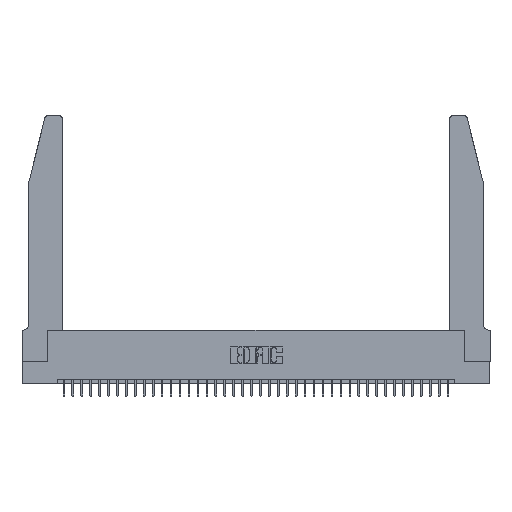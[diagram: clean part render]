
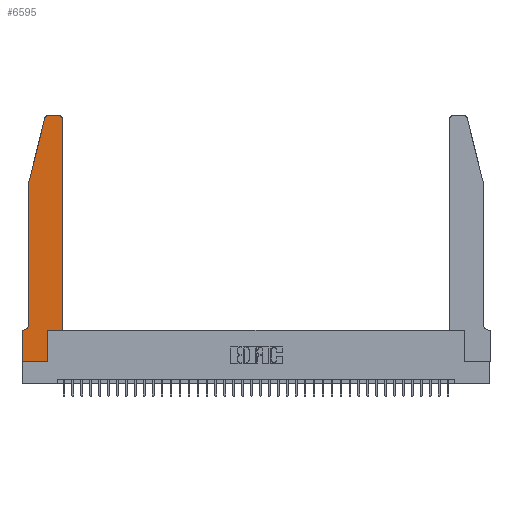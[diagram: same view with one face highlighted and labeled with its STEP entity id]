
A CAD part, top view. The second image highlights one B-rep face of the part: STEP entity #6595.
In plain terms, the highlighted planar face has unit normal (0, 0, 1).
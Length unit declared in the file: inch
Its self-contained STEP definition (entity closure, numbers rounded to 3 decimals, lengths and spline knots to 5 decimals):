
#118 = CARTESIAN_POINT ( 'NONE',  ( 0.2865, 0., 0.37 ) ) ;
#258 = EDGE_CURVE ( 'NONE', #8213, #38818, #25782, .T. ) ;
#737 = EDGE_CURVE ( 'NONE', #27138, #36192, #26523, .T. ) ;
#896 = DIRECTION ( 'NONE',  ( 0., 1., 0. ) ) ;
#1675 = DIRECTION ( 'NONE',  ( -1., 0., 0. ) ) ;
#2012 = CARTESIAN_POINT ( 'NONE',  ( 0.4505, 0.35, 0.37 ) ) ;
#2099 = CARTESIAN_POINT ( 'NONE',  ( 0.4205, 2.75, 0.37 ) ) ;
#3438 = AXIS2_PLACEMENT_3D ( 'NONE', #30439, #6475, #11615 ) ;
#3980 = DIRECTION ( 'NONE',  ( -1., 0., 0. ) ) ;
#4992 = EDGE_LOOP ( 'NONE', ( #22678, #20300, #11298, #25107, #38642, #12023, #14114, #24046, #18698, #20896, #29442, #15454 ) ) ;
#5937 = CIRCLE ( 'NONE', #3438, 0.03 ) ;
#6475 = DIRECTION ( 'NONE',  ( 0., 0., 1. ) ) ;
#6574 = DIRECTION ( 'NONE',  ( 0., 1., 0. ) ) ;
#6595 = ADVANCED_FACE ( 'NONE', ( #8096 ), #20915, .T. ) ;
#6707 = VERTEX_POINT ( 'NONE', #21108 ) ;
#6776 = CARTESIAN_POINT ( 'NONE',  ( 0.0055, 0.42, 0.37 ) ) ;
#6974 = DIRECTION ( 'NONE',  ( 0., 0., 1. ) ) ;
#7736 = VECTOR ( 'NONE', #33740, 39.37008 ) ;
#8096 = FACE_OUTER_BOUND ( 'NONE', #4992, .T. ) ;
#8213 = VERTEX_POINT ( 'NONE', #11500 ) ;
#8714 = CARTESIAN_POINT ( 'NONE',  ( 0., 0.35, 0.37 ) ) ;
#8911 = EDGE_CURVE ( 'NONE', #25903, #9559, #16449, .T. ) ;
#9214 = LINE ( 'NONE', #15298, #7736 ) ;
#9313 = CARTESIAN_POINT ( 'NONE',  ( 0.0755, 0.35, 0.37 ) ) ;
#9559 = VERTEX_POINT ( 'NONE', #15037 ) ;
#9956 = CARTESIAN_POINT ( 'NONE',  ( 0.284, 2.72, 0.37 ) ) ;
#10359 = CARTESIAN_POINT ( 'NONE',  ( 0.2865, 0.35, 0.37 ) ) ;
#10365 = VERTEX_POINT ( 'NONE', #38243 ) ;
#10992 = CARTESIAN_POINT ( 'NONE',  ( 0.4505, 2.72, 0.37 ) ) ;
#11298 = ORIENTED_EDGE ( 'NONE', *, *, #29453, .T. ) ;
#11379 = VECTOR ( 'NONE', #32501, 39.37008 ) ;
#11500 = CARTESIAN_POINT ( 'NONE',  ( 0.2865, 0.35, 0.37 ) ) ;
#11615 = DIRECTION ( 'NONE',  ( 1., 0., 0. ) ) ;
#11688 = CIRCLE ( 'NONE', #23052, 0.07 ) ;
#12023 = ORIENTED_EDGE ( 'NONE', *, *, #737, .T. ) ;
#13085 = EDGE_CURVE ( 'NONE', #20091, #8213, #27633, .T. ) ;
#13497 = AXIS2_PLACEMENT_3D ( 'NONE', #9956, #6974, #28169 ) ;
#14114 = ORIENTED_EDGE ( 'NONE', *, *, #36691, .T. ) ;
#15037 = CARTESIAN_POINT ( 'NONE',  ( 0.284, 2.75, 0.37 ) ) ;
#15298 = CARTESIAN_POINT ( 'NONE',  ( 0., 0., 0.37 ) ) ;
#15349 = EDGE_CURVE ( 'NONE', #6707, #10365, #28744, .T. ) ;
#15454 = ORIENTED_EDGE ( 'NONE', *, *, #28940, .T. ) ;
#16449 = LINE ( 'NONE', #25426, #30120 ) ;
#17530 = CARTESIAN_POINT ( 'NONE',  ( 0.25487, 2.72718, 0.37 ) ) ;
#18368 = CARTESIAN_POINT ( 'NONE',  ( 0., 0., 0.37 ) ) ;
#18423 = CARTESIAN_POINT ( 'NONE',  ( 0.4505, 0.35, 0.37 ) ) ;
#18698 = ORIENTED_EDGE ( 'NONE', *, *, #13085, .T. ) ;
#19200 = CIRCLE ( 'NONE', #13497, 0.03 ) ;
#20091 = VERTEX_POINT ( 'NONE', #118 ) ;
#20300 = ORIENTED_EDGE ( 'NONE', *, *, #27486, .T. ) ;
#20401 = VECTOR ( 'NONE', #6574, 39.37008 ) ;
#20813 = VECTOR ( 'NONE', #896, 39.37008 ) ;
#20896 = ORIENTED_EDGE ( 'NONE', *, *, #258, .T. ) ;
#20915 = PLANE ( 'NONE',  #31883 ) ;
#21108 = CARTESIAN_POINT ( 'NONE',  ( 0.0755, 2., 0.37 ) ) ;
#22195 = CARTESIAN_POINT ( 'NONE',  ( 0.0755, 2., 0.37 ) ) ;
#22678 = ORIENTED_EDGE ( 'NONE', *, *, #8911, .T. ) ;
#23052 = AXIS2_PLACEMENT_3D ( 'NONE', #6776, #31117, #3980 ) ;
#23770 = LINE ( 'NONE', #18368, #35732 ) ;
#23858 = VERTEX_POINT ( 'NONE', #10992 ) ;
#24046 = ORIENTED_EDGE ( 'NONE', *, *, #28577, .T. ) ;
#24059 = DIRECTION ( 'NONE',  ( -0.239, -0.971, 0. ) ) ;
#24858 = CARTESIAN_POINT ( 'NONE',  ( 0.0055, 0.35, 0.37 ) ) ;
#25107 = ORIENTED_EDGE ( 'NONE', *, *, #15349, .T. ) ;
#25426 = CARTESIAN_POINT ( 'NONE',  ( 0.2605, 2.75, 0.37 ) ) ;
#25782 = LINE ( 'NONE', #2012, #11379 ) ;
#25903 = VERTEX_POINT ( 'NONE', #2099 ) ;
#25985 = VECTOR ( 'NONE', #29893, 39.37008 ) ;
#26523 = LINE ( 'NONE', #9313, #25985 ) ;
#27138 = VERTEX_POINT ( 'NONE', #24858 ) ;
#27428 = LINE ( 'NONE', #32774, #35701 ) ;
#27486 = EDGE_CURVE ( 'NONE', #9559, #27837, #19200, .T. ) ;
#27633 = LINE ( 'NONE', #10359, #20813 ) ;
#27837 = VERTEX_POINT ( 'NONE', #17530 ) ;
#28169 = DIRECTION ( 'NONE',  ( 1., 0., 0. ) ) ;
#28577 = EDGE_CURVE ( 'NONE', #36364, #20091, #23770, .T. ) ;
#28744 = LINE ( 'NONE', #22195, #32016 ) ;
#28940 = EDGE_CURVE ( 'NONE', #23858, #25903, #5937, .T. ) ;
#29442 = ORIENTED_EDGE ( 'NONE', *, *, #35426, .T. ) ;
#29453 = EDGE_CURVE ( 'NONE', #27837, #6707, #27428, .T. ) ;
#29472 = DIRECTION ( 'NONE',  ( 0., 0., 1. ) ) ;
#29864 = CARTESIAN_POINT ( 'NONE',  ( 0.4505, 0.35, 0.37 ) ) ;
#29893 = DIRECTION ( 'NONE',  ( -1., 0., 0. ) ) ;
#29911 = DIRECTION ( 'NONE',  ( 1., 0., 0. ) ) ;
#29989 = EDGE_CURVE ( 'NONE', #10365, #27138, #11688, .T. ) ;
#30120 = VECTOR ( 'NONE', #1675, 39.37008 ) ;
#30439 = CARTESIAN_POINT ( 'NONE',  ( 0.4205, 2.72, 0.37 ) ) ;
#30829 = CARTESIAN_POINT ( 'NONE',  ( 0., 0., 0.37 ) ) ;
#31117 = DIRECTION ( 'NONE',  ( 0., 0., -1. ) ) ;
#31883 = AXIS2_PLACEMENT_3D ( 'NONE', #8714, #29472, #33019 ) ;
#32016 = VECTOR ( 'NONE', #34288, 39.37008 ) ;
#32501 = DIRECTION ( 'NONE',  ( 1., 0., 0. ) ) ;
#32609 = CARTESIAN_POINT ( 'NONE',  ( 0., 0.35, 0.37 ) ) ;
#32774 = CARTESIAN_POINT ( 'NONE',  ( 0.0755, 2., 0.37 ) ) ;
#33019 = DIRECTION ( 'NONE',  ( 1., 0., 0. ) ) ;
#33501 = LINE ( 'NONE', #18423, #20401 ) ;
#33740 = DIRECTION ( 'NONE',  ( 0., -1., 0. ) ) ;
#34288 = DIRECTION ( 'NONE',  ( 0., -1., 0. ) ) ;
#35426 = EDGE_CURVE ( 'NONE', #38818, #23858, #33501, .T. ) ;
#35701 = VECTOR ( 'NONE', #24059, 39.37008 ) ;
#35732 = VECTOR ( 'NONE', #29911, 39.37008 ) ;
#36192 = VERTEX_POINT ( 'NONE', #32609 ) ;
#36364 = VERTEX_POINT ( 'NONE', #30829 ) ;
#36691 = EDGE_CURVE ( 'NONE', #36192, #36364, #9214, .T. ) ;
#38243 = CARTESIAN_POINT ( 'NONE',  ( 0.0755, 0.42, 0.37 ) ) ;
#38642 = ORIENTED_EDGE ( 'NONE', *, *, #29989, .T. ) ;
#38818 = VERTEX_POINT ( 'NONE', #29864 ) ;
